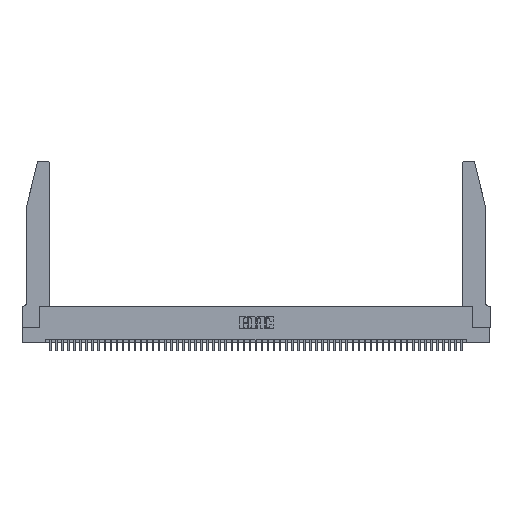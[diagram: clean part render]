
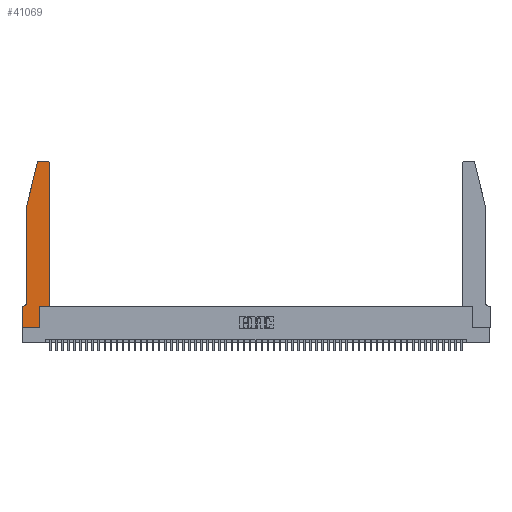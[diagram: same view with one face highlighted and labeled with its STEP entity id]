
A CAD part, top view. The second image highlights one B-rep face of the part: STEP entity #41069.
In plain terms, the highlighted planar face has unit normal (0, 0, 1).
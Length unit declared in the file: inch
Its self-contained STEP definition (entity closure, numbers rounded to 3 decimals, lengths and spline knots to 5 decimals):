
#2803 = ORIENTED_EDGE ( 'NONE', *, *, #36053, .T. ) ;
#3283 = CARTESIAN_POINT ( 'NONE',  ( 0.2865, 0.35, 0.37 ) ) ;
#3721 = AXIS2_PLACEMENT_3D ( 'NONE', #42053, #50585, #12124 ) ;
#3918 = VERTEX_POINT ( 'NONE', #3283 ) ;
#4164 = DIRECTION ( 'NONE',  ( -0.239, -0.971, 0. ) ) ;
#4441 = EDGE_CURVE ( 'NONE', #6155, #43187, #44741, .T. ) ;
#4886 = VECTOR ( 'NONE', #4164, 39.37008 ) ;
#5176 = EDGE_CURVE ( 'NONE', #24714, #43215, #8537, .T. ) ;
#5717 = CARTESIAN_POINT ( 'NONE',  ( 0., 0., 0.37 ) ) ;
#6155 = VERTEX_POINT ( 'NONE', #27329 ) ;
#6163 = DIRECTION ( 'NONE',  ( 0., 0., 1. ) ) ;
#6387 = DIRECTION ( 'NONE',  ( -1., 0., 0. ) ) ;
#6437 = LINE ( 'NONE', #49663, #11096 ) ;
#7274 = DIRECTION ( 'NONE',  ( 0., 1., 0. ) ) ;
#7303 = VECTOR ( 'NONE', #32750, 39.37008 ) ;
#7616 = ORIENTED_EDGE ( 'NONE', *, *, #18104, .T. ) ;
#8537 = LINE ( 'NONE', #15321, #49325 ) ;
#9549 = LINE ( 'NONE', #21163, #4886 ) ;
#9984 = DIRECTION ( 'NONE',  ( 1., 0., 0. ) ) ;
#11096 = VECTOR ( 'NONE', #40756, 39.37008 ) ;
#11110 = CARTESIAN_POINT ( 'NONE',  ( 0.2865, 0., 0.37 ) ) ;
#11724 = EDGE_CURVE ( 'NONE', #43187, #3918, #36010, .T. ) ;
#12124 = DIRECTION ( 'NONE',  ( -1., 0., 0. ) ) ;
#12269 = ORIENTED_EDGE ( 'NONE', *, *, #15920, .T. ) ;
#12754 = CARTESIAN_POINT ( 'NONE',  ( 0.284, 2.75, 0.37 ) ) ;
#13809 = LINE ( 'NONE', #18038, #15838 ) ;
#15321 = CARTESIAN_POINT ( 'NONE',  ( 0.4505, 0.35, 0.37 ) ) ;
#15471 = ORIENTED_EDGE ( 'NONE', *, *, #53512, .T. ) ;
#15838 = VECTOR ( 'NONE', #38633, 39.37008 ) ;
#15920 = EDGE_CURVE ( 'NONE', #34034, #17489, #28108, .T. ) ;
#16699 = EDGE_CURVE ( 'NONE', #17489, #6155, #27439, .T. ) ;
#17489 = VERTEX_POINT ( 'NONE', #23053 ) ;
#18038 = CARTESIAN_POINT ( 'NONE',  ( 0.0755, 2., 0.37 ) ) ;
#18104 = EDGE_CURVE ( 'NONE', #43215, #37049, #19979, .T. ) ;
#18502 = CARTESIAN_POINT ( 'NONE',  ( 0.0755, 0.35, 0.37 ) ) ;
#19393 = ORIENTED_EDGE ( 'NONE', *, *, #38029, .T. ) ;
#19979 = CIRCLE ( 'NONE', #21894, 0.03 ) ;
#21163 = CARTESIAN_POINT ( 'NONE',  ( 0.0755, 2., 0.37 ) ) ;
#21254 = CARTESIAN_POINT ( 'NONE',  ( 0.284, 2.72, 0.37 ) ) ;
#21894 = AXIS2_PLACEMENT_3D ( 'NONE', #31560, #6163, #26909 ) ;
#21952 = EDGE_CURVE ( 'NONE', #28066, #42033, #9549, .T. ) ;
#22353 = LINE ( 'NONE', #52704, #41808 ) ;
#22501 = DIRECTION ( 'NONE',  ( 0., 0., 1. ) ) ;
#23053 = CARTESIAN_POINT ( 'NONE',  ( 0., 0.35, 0.37 ) ) ;
#23125 = ORIENTED_EDGE ( 'NONE', *, *, #16699, .T. ) ;
#24636 = VECTOR ( 'NONE', #29577, 39.37008 ) ;
#24714 = VERTEX_POINT ( 'NONE', #51011 ) ;
#25231 = EDGE_LOOP ( 'NONE', ( #25479, #15471, #41510, #19393, #38309, #12269, #23125, #33879, #48441, #2803, #45577, #7616 ) ) ;
#25479 = ORIENTED_EDGE ( 'NONE', *, *, #38930, .T. ) ;
#26102 = VECTOR ( 'NONE', #27097, 39.37008 ) ;
#26909 = DIRECTION ( 'NONE',  ( 1., 0., 0. ) ) ;
#27097 = DIRECTION ( 'NONE',  ( -1., 0., 0. ) ) ;
#27329 = CARTESIAN_POINT ( 'NONE',  ( 0., 0., 0.37 ) ) ;
#27364 = CARTESIAN_POINT ( 'NONE',  ( 0., 0.35, 0.37 ) ) ;
#27439 = LINE ( 'NONE', #5717, #50146 ) ;
#28066 = VERTEX_POINT ( 'NONE', #45893 ) ;
#28108 = LINE ( 'NONE', #18502, #26102 ) ;
#28226 = VERTEX_POINT ( 'NONE', #43437 ) ;
#29577 = DIRECTION ( 'NONE',  ( 0., 1., 0. ) ) ;
#31560 = CARTESIAN_POINT ( 'NONE',  ( 0.4205, 2.72, 0.37 ) ) ;
#32750 = DIRECTION ( 'NONE',  ( 1., 0., 0. ) ) ;
#33150 = CARTESIAN_POINT ( 'NONE',  ( 0.4505, 2.72, 0.37 ) ) ;
#33879 = ORIENTED_EDGE ( 'NONE', *, *, #4441, .T. ) ;
#34034 = VERTEX_POINT ( 'NONE', #54384 ) ;
#34183 = VERTEX_POINT ( 'NONE', #12754 ) ;
#35258 = DIRECTION ( 'NONE',  ( 0., -1., 0. ) ) ;
#36010 = LINE ( 'NONE', #55171, #24636 ) ;
#36053 = EDGE_CURVE ( 'NONE', #3918, #24714, #6437, .T. ) ;
#36877 = AXIS2_PLACEMENT_3D ( 'NONE', #27364, #22501, #9984 ) ;
#37049 = VERTEX_POINT ( 'NONE', #42888 ) ;
#38029 = EDGE_CURVE ( 'NONE', #42033, #28226, #13809, .T. ) ;
#38309 = ORIENTED_EDGE ( 'NONE', *, *, #47287, .T. ) ;
#38633 = DIRECTION ( 'NONE',  ( 0., -1., 0. ) ) ;
#38930 = EDGE_CURVE ( 'NONE', #37049, #34183, #22353, .T. ) ;
#40756 = DIRECTION ( 'NONE',  ( 1., 0., 0. ) ) ;
#41069 = ADVANCED_FACE ( 'NONE', ( #44951 ), #48671, .T. ) ;
#41510 = ORIENTED_EDGE ( 'NONE', *, *, #21952, .T. ) ;
#41808 = VECTOR ( 'NONE', #6387, 39.37008 ) ;
#42033 = VERTEX_POINT ( 'NONE', #53970 ) ;
#42053 = CARTESIAN_POINT ( 'NONE',  ( 0.0055, 0.42, 0.37 ) ) ;
#42888 = CARTESIAN_POINT ( 'NONE',  ( 0.4205, 2.75, 0.37 ) ) ;
#43187 = VERTEX_POINT ( 'NONE', #11110 ) ;
#43215 = VERTEX_POINT ( 'NONE', #33150 ) ;
#43437 = CARTESIAN_POINT ( 'NONE',  ( 0.0755, 0.42, 0.37 ) ) ;
#44358 = CIRCLE ( 'NONE', #51102, 0.03 ) ;
#44741 = LINE ( 'NONE', #54197, #7303 ) ;
#44951 = FACE_OUTER_BOUND ( 'NONE', #25231, .T. ) ;
#45577 = ORIENTED_EDGE ( 'NONE', *, *, #5176, .T. ) ;
#45893 = CARTESIAN_POINT ( 'NONE',  ( 0.25487, 2.72718, 0.37 ) ) ;
#47287 = EDGE_CURVE ( 'NONE', #28226, #34034, #51743, .T. ) ;
#48441 = ORIENTED_EDGE ( 'NONE', *, *, #11724, .T. ) ;
#48671 = PLANE ( 'NONE',  #36877 ) ;
#49325 = VECTOR ( 'NONE', #7274, 39.37008 ) ;
#49663 = CARTESIAN_POINT ( 'NONE',  ( 0.4505, 0.35, 0.37 ) ) ;
#50146 = VECTOR ( 'NONE', #35258, 39.37008 ) ;
#50585 = DIRECTION ( 'NONE',  ( 0., 0., -1. ) ) ;
#51011 = CARTESIAN_POINT ( 'NONE',  ( 0.4505, 0.35, 0.37 ) ) ;
#51102 = AXIS2_PLACEMENT_3D ( 'NONE', #21254, #51312, #55227 ) ;
#51312 = DIRECTION ( 'NONE',  ( 0., 0., 1. ) ) ;
#51743 = CIRCLE ( 'NONE', #3721, 0.07 ) ;
#52704 = CARTESIAN_POINT ( 'NONE',  ( 0.2605, 2.75, 0.37 ) ) ;
#53512 = EDGE_CURVE ( 'NONE', #34183, #28066, #44358, .T. ) ;
#53970 = CARTESIAN_POINT ( 'NONE',  ( 0.0755, 2., 0.37 ) ) ;
#54197 = CARTESIAN_POINT ( 'NONE',  ( 0., 0., 0.37 ) ) ;
#54384 = CARTESIAN_POINT ( 'NONE',  ( 0.0055, 0.35, 0.37 ) ) ;
#55171 = CARTESIAN_POINT ( 'NONE',  ( 0.2865, 0.35, 0.37 ) ) ;
#55227 = DIRECTION ( 'NONE',  ( 1., 0., 0. ) ) ;
